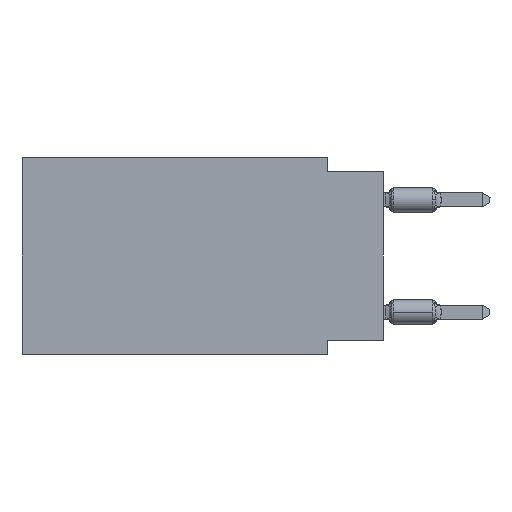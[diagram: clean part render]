
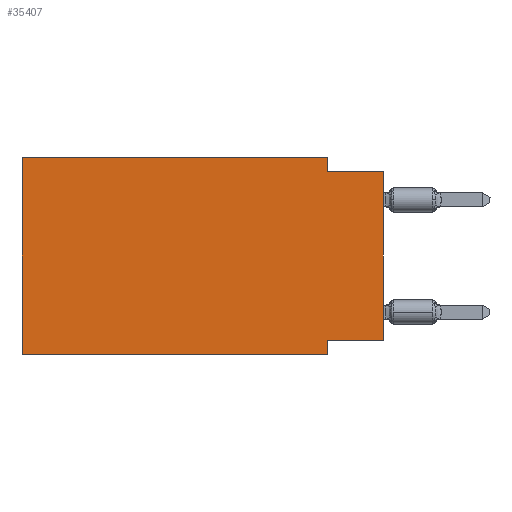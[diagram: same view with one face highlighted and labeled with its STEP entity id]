
A CAD part, left-side view. The second image highlights one B-rep face of the part: STEP entity #35407.
In plain terms, the highlighted planar face has unit normal (-1, 0, 0).
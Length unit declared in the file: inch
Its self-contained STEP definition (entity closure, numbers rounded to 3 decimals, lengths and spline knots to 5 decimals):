
#830 = DIRECTION ( 'NONE',  ( 0., -1., 0. ) ) ;
#1933 = CARTESIAN_POINT ( 'NONE',  ( 0., 0.1, -0.35 ) ) ;
#3689 = VECTOR ( 'NONE', #19408, 39.37008 ) ;
#5440 = VERTEX_POINT ( 'NONE', #15570 ) ;
#5824 = ORIENTED_EDGE ( 'NONE', *, *, #55938, .F. ) ;
#7655 = CARTESIAN_POINT ( 'NONE',  ( 0., 0.645, 0. ) ) ;
#8086 = VERTEX_POINT ( 'NONE', #59795 ) ;
#8939 = EDGE_CURVE ( 'NONE', #8086, #11806, #34012, .T. ) ;
#10096 = VERTEX_POINT ( 'NONE', #44464 ) ;
#10456 = DIRECTION ( 'NONE',  ( 1., 0., 0. ) ) ;
#10837 = ORIENTED_EDGE ( 'NONE', *, *, #34667, .T. ) ;
#11012 = LINE ( 'NONE', #25620, #55589 ) ;
#11488 = EDGE_CURVE ( 'NONE', #14837, #30691, #33249, .T. ) ;
#11806 = VERTEX_POINT ( 'NONE', #36187 ) ;
#11812 = EDGE_CURVE ( 'NONE', #5440, #10096, #56152, .T. ) ;
#14477 = ORIENTED_EDGE ( 'NONE', *, *, #8939, .F. ) ;
#14794 = CARTESIAN_POINT ( 'NONE',  ( 0., 0., -0.325 ) ) ;
#14837 = VERTEX_POINT ( 'NONE', #47414 ) ;
#15570 = CARTESIAN_POINT ( 'NONE',  ( 0., 0.1, -0.325 ) ) ;
#16034 = CARTESIAN_POINT ( 'NONE',  ( 0., 0., -0.325 ) ) ;
#16576 = VECTOR ( 'NONE', #40059, 39.37008 ) ;
#19408 = DIRECTION ( 'NONE',  ( 0., 0., -1. ) ) ;
#19873 = EDGE_LOOP ( 'NONE', ( #10837, #5824, #14477, #30381, #42495, #51726, #37029, #22641 ) ) ;
#20817 = CARTESIAN_POINT ( 'NONE',  ( 0., 0.645, 0. ) ) ;
#21580 = DIRECTION ( 'NONE',  ( 0., 0., -1. ) ) ;
#21792 = LINE ( 'NONE', #20817, #48114 ) ;
#22641 = ORIENTED_EDGE ( 'NONE', *, *, #31581, .F. ) ;
#24767 = LINE ( 'NONE', #14794, #16576 ) ;
#25474 = DIRECTION ( 'NONE',  ( 0., 0., 1. ) ) ;
#25604 = AXIS2_PLACEMENT_3D ( 'NONE', #26082, #10456, #41701 ) ;
#25620 = CARTESIAN_POINT ( 'NONE',  ( 0., 0., -0.025 ) ) ;
#26082 = CARTESIAN_POINT ( 'NONE',  ( 0., 0.645, 0. ) ) ;
#26410 = VERTEX_POINT ( 'NONE', #16034 ) ;
#30381 = ORIENTED_EDGE ( 'NONE', *, *, #38808, .F. ) ;
#30612 = DIRECTION ( 'NONE',  ( 0., -1., 0. ) ) ;
#30691 = VERTEX_POINT ( 'NONE', #54050 ) ;
#31581 = EDGE_CURVE ( 'NONE', #26410, #5440, #24767, .T. ) ;
#33249 = LINE ( 'NONE', #7655, #62248 ) ;
#34012 = LINE ( 'NONE', #44660, #3689 ) ;
#34038 = VECTOR ( 'NONE', #25474, 39.37008 ) ;
#34667 = EDGE_CURVE ( 'NONE', #26410, #61209, #60415, .T. ) ;
#35407 = ADVANCED_FACE ( 'NONE', ( #36381 ), #51359, .F. ) ;
#35684 = VECTOR ( 'NONE', #21580, 39.37008 ) ;
#36049 = DIRECTION ( 'NONE',  ( 0., -1., 0. ) ) ;
#36187 = CARTESIAN_POINT ( 'NONE',  ( 0., 0.1, -0.025 ) ) ;
#36381 = FACE_OUTER_BOUND ( 'NONE', #19873, .T. ) ;
#36645 = EDGE_CURVE ( 'NONE', #14837, #10096, #50710, .T. ) ;
#37029 = ORIENTED_EDGE ( 'NONE', *, *, #11812, .F. ) ;
#37267 = VECTOR ( 'NONE', #36049, 39.37008 ) ;
#38808 = EDGE_CURVE ( 'NONE', #30691, #8086, #21792, .T. ) ;
#40059 = DIRECTION ( 'NONE',  ( 0., 1., 0. ) ) ;
#40519 = CARTESIAN_POINT ( 'NONE',  ( 0., 0., -0.025 ) ) ;
#41701 = DIRECTION ( 'NONE',  ( 0., 0., -1. ) ) ;
#42495 = ORIENTED_EDGE ( 'NONE', *, *, #11488, .F. ) ;
#43893 = DIRECTION ( 'NONE',  ( 0., 0., 1. ) ) ;
#44464 = CARTESIAN_POINT ( 'NONE',  ( 0., 0.1, -0.35 ) ) ;
#44660 = CARTESIAN_POINT ( 'NONE',  ( 0., 0.1, 0. ) ) ;
#46381 = CARTESIAN_POINT ( 'NONE',  ( 0., 0.645, -0.35 ) ) ;
#47414 = CARTESIAN_POINT ( 'NONE',  ( 0., 0.645, -0.35 ) ) ;
#48114 = VECTOR ( 'NONE', #830, 39.37008 ) ;
#50710 = LINE ( 'NONE', #46381, #37267 ) ;
#51359 = PLANE ( 'NONE',  #25604 ) ;
#51726 = ORIENTED_EDGE ( 'NONE', *, *, #36645, .T. ) ;
#54050 = CARTESIAN_POINT ( 'NONE',  ( 0., 0.645, 0. ) ) ;
#55589 = VECTOR ( 'NONE', #30612, 39.37008 ) ;
#55752 = CARTESIAN_POINT ( 'NONE',  ( 0., 0., 0. ) ) ;
#55938 = EDGE_CURVE ( 'NONE', #11806, #61209, #11012, .T. ) ;
#56152 = LINE ( 'NONE', #1933, #35684 ) ;
#59795 = CARTESIAN_POINT ( 'NONE',  ( 0., 0.1, 0. ) ) ;
#60415 = LINE ( 'NONE', #55752, #34038 ) ;
#61209 = VERTEX_POINT ( 'NONE', #40519 ) ;
#62248 = VECTOR ( 'NONE', #43893, 39.37008 ) ;
